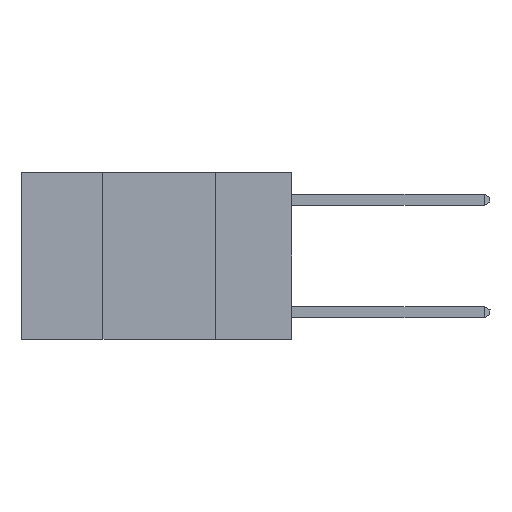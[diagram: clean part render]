
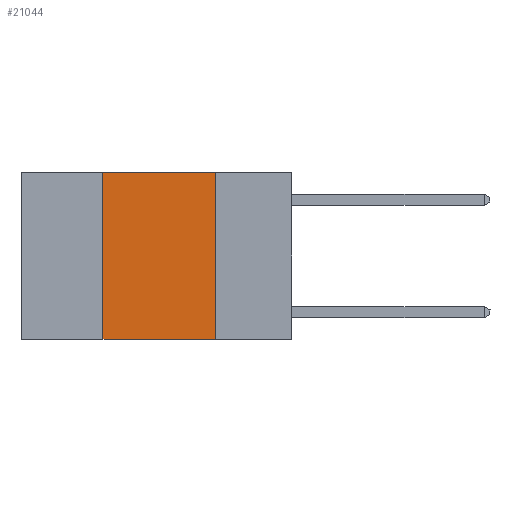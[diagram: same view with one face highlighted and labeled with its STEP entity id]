
A CAD part, left-side view. The second image highlights one B-rep face of the part: STEP entity #21044.
In plain terms, the highlighted planar face has unit normal (-1, 0, 0).
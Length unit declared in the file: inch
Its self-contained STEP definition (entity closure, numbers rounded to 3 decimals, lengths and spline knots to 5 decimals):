
#280 = EDGE_CURVE ( 'NONE', #17198, #24217, #1986, .T. ) ;
#1132 = DIRECTION ( 'NONE',  ( 0., 0., -1. ) ) ;
#1288 = CARTESIAN_POINT ( 'NONE',  ( 0., 0.17, -0.37 ) ) ;
#1986 = LINE ( 'NONE', #7165, #16684 ) ;
#3457 = VECTOR ( 'NONE', #13707, 39.37008 ) ;
#3591 = EDGE_CURVE ( 'NONE', #5164, #8534, #13678, .T. ) ;
#4709 = EDGE_CURVE ( 'NONE', #8534, #24217, #19449, .T. ) ;
#5003 = PLANE ( 'NONE',  #8346 ) ;
#5164 = VERTEX_POINT ( 'NONE', #21520 ) ;
#5295 = LINE ( 'NONE', #6589, #19787 ) ;
#5554 = DIRECTION ( 'NONE',  ( 0., -1., 0. ) ) ;
#5709 = ORIENTED_EDGE ( 'NONE', *, *, #4709, .F. ) ;
#5746 = FACE_OUTER_BOUND ( 'NONE', #6300, .T. ) ;
#6300 = EDGE_LOOP ( 'NONE', ( #5709, #12691, #17683, #21328 ) ) ;
#6589 = CARTESIAN_POINT ( 'NONE',  ( 0., 0.42, 0. ) ) ;
#7165 = CARTESIAN_POINT ( 'NONE',  ( 0., 0.6, -0.37 ) ) ;
#8346 = AXIS2_PLACEMENT_3D ( 'NONE', #23770, #12711, #1132 ) ;
#8534 = VERTEX_POINT ( 'NONE', #12749 ) ;
#11207 = CARTESIAN_POINT ( 'NONE',  ( 0., 0.42, -0.37 ) ) ;
#12691 = ORIENTED_EDGE ( 'NONE', *, *, #3591, .F. ) ;
#12711 = DIRECTION ( 'NONE',  ( 1., 0., 0. ) ) ;
#12749 = CARTESIAN_POINT ( 'NONE',  ( 0., 0.17, 0. ) ) ;
#12927 = DIRECTION ( 'NONE',  ( 0., 0., -1. ) ) ;
#13678 = LINE ( 'NONE', #15592, #3457 ) ;
#13707 = DIRECTION ( 'NONE',  ( 0., -1., 0. ) ) ;
#14259 = DIRECTION ( 'NONE',  ( 0., 0., 1. ) ) ;
#15106 = VECTOR ( 'NONE', #12927, 39.37008 ) ;
#15592 = CARTESIAN_POINT ( 'NONE',  ( 0., 0.6, 0. ) ) ;
#16684 = VECTOR ( 'NONE', #5554, 39.37008 ) ;
#17198 = VERTEX_POINT ( 'NONE', #11207 ) ;
#17683 = ORIENTED_EDGE ( 'NONE', *, *, #24045, .F. ) ;
#19449 = LINE ( 'NONE', #23977, #15106 ) ;
#19787 = VECTOR ( 'NONE', #14259, 39.37008 ) ;
#21044 = ADVANCED_FACE ( 'NONE', ( #5746 ), #5003, .F. ) ;
#21328 = ORIENTED_EDGE ( 'NONE', *, *, #280, .T. ) ;
#21520 = CARTESIAN_POINT ( 'NONE',  ( 0., 0.42, 0. ) ) ;
#23770 = CARTESIAN_POINT ( 'NONE',  ( 0., 0.6, 0. ) ) ;
#23977 = CARTESIAN_POINT ( 'NONE',  ( 0., 0.17, 0. ) ) ;
#24045 = EDGE_CURVE ( 'NONE', #17198, #5164, #5295, .T. ) ;
#24217 = VERTEX_POINT ( 'NONE', #1288 ) ;
